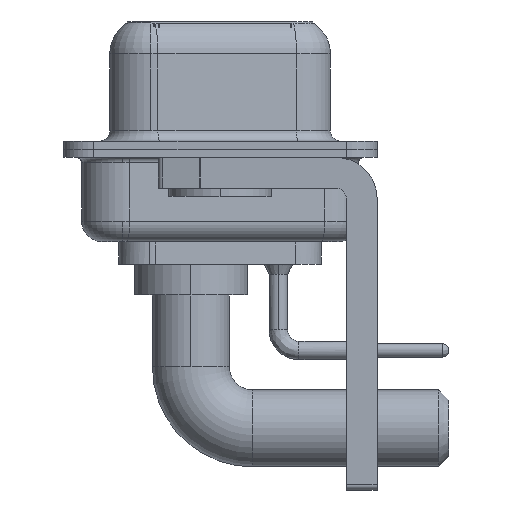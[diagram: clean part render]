
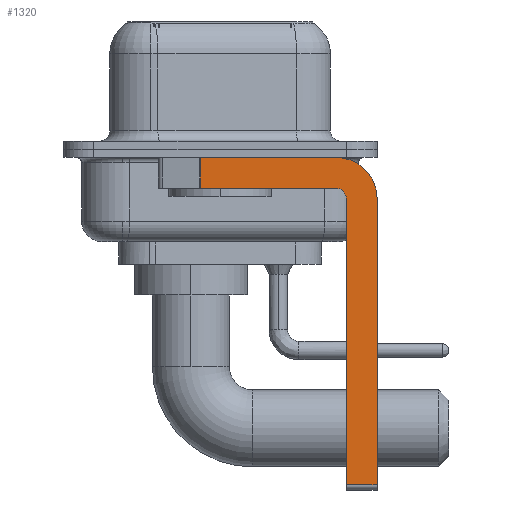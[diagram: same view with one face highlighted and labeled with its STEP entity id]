
A CAD part, left-side view. The second image highlights one B-rep face of the part: STEP entity #1320.
In plain terms, the highlighted planar face has unit normal (-1, 0, 0).
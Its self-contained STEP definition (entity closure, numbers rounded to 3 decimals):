
#208 = CARTESIAN_POINT ( 'NONE',  ( -2.9, 3., -0.4 ) ) ;
#1047 = AXIS2_PLACEMENT_3D ( 'NONE', #15279, #2071, #10603 ) ;
#1320 = ADVANCED_FACE ( 'NONE', ( #20540 ), #8215, .F. ) ;
#1343 = EDGE_CURVE ( 'NONE', #2158, #10176, #16879, .T. ) ;
#1547 = CARTESIAN_POINT ( 'NONE',  ( -2.9, -5.65, -2.4 ) ) ;
#1676 = DIRECTION ( 'NONE',  ( 0., -1., 0. ) ) ;
#2071 = DIRECTION ( 'NONE',  ( 1., 0., 0. ) ) ;
#2158 = VERTEX_POINT ( 'NONE', #21906 ) ;
#2584 = DIRECTION ( 'NONE',  ( 0., -1., 0. ) ) ;
#2932 = CARTESIAN_POINT ( 'NONE',  ( -2.9, -6.15, -2.4 ) ) ;
#2964 = CARTESIAN_POINT ( 'NONE',  ( -2.9, 0.978, -1.9 ) ) ;
#2982 = CARTESIAN_POINT ( 'NONE',  ( -2.9, 0.978, -1.9 ) ) ;
#3228 = VERTEX_POINT ( 'NONE', #15594 ) ;
#3400 = ORIENTED_EDGE ( 'NONE', *, *, #13802, .F. ) ;
#3750 = AXIS2_PLACEMENT_3D ( 'NONE', #1547, #20100, #18533 ) ;
#3889 = VECTOR ( 'NONE', #2584, 1000. ) ;
#4339 = VECTOR ( 'NONE', #12668, 1000. ) ;
#4344 = CARTESIAN_POINT ( 'NONE',  ( -2.9, -5.65, -1.9 ) ) ;
#4387 = VECTOR ( 'NONE', #21651, 1000. ) ;
#4644 = CARTESIAN_POINT ( 'NONE',  ( -2.9, -7.65, -2.4 ) ) ;
#4808 = ORIENTED_EDGE ( 'NONE', *, *, #9100, .F. ) ;
#4997 = CARTESIAN_POINT ( 'NONE',  ( -2.9, -5.65, -2.4 ) ) ;
#5145 = EDGE_CURVE ( 'NONE', #15355, #3228, #19470, .T. ) ;
#5320 = DIRECTION ( 'NONE',  ( 0., 0., -1. ) ) ;
#5697 = ORIENTED_EDGE ( 'NONE', *, *, #19944, .F. ) ;
#5735 = ORIENTED_EDGE ( 'NONE', *, *, #8685, .F. ) ;
#6081 = CARTESIAN_POINT ( 'NONE',  ( -2.9, -6.15, -16.35 ) ) ;
#6091 = VECTOR ( 'NONE', #7573, 1000. ) ;
#6569 = CARTESIAN_POINT ( 'NONE',  ( -2.9, -5.65, -0.4 ) ) ;
#6638 = VECTOR ( 'NONE', #1676, 1000. ) ;
#6986 = VERTEX_POINT ( 'NONE', #4344 ) ;
#7358 = LINE ( 'NONE', #4644, #6091 ) ;
#7573 = DIRECTION ( 'NONE',  ( 0., 0., -1. ) ) ;
#8215 = PLANE ( 'NONE',  #15480 ) ;
#8685 = EDGE_CURVE ( 'NONE', #10845, #3228, #7358, .T. ) ;
#9100 = EDGE_CURVE ( 'NONE', #15355, #11179, #9284, .T. ) ;
#9210 = LINE ( 'NONE', #15990, #4339 ) ;
#9284 = LINE ( 'NONE', #16064, #19599 ) ;
#10176 = VERTEX_POINT ( 'NONE', #6569 ) ;
#10603 = DIRECTION ( 'NONE',  ( 0., 0., -1. ) ) ;
#10845 = VERTEX_POINT ( 'NONE', #18503 ) ;
#11179 = VERTEX_POINT ( 'NONE', #2932 ) ;
#12248 = ORIENTED_EDGE ( 'NONE', *, *, #15546, .F. ) ;
#12668 = DIRECTION ( 'NONE',  ( 0., 1., 0. ) ) ;
#13802 = EDGE_CURVE ( 'NONE', #11179, #6986, #20790, .T. ) ;
#14986 = DIRECTION ( 'NONE',  ( 1., 0., 0. ) ) ;
#15279 = CARTESIAN_POINT ( 'NONE',  ( -2.9, -5.65, -2.4 ) ) ;
#15355 = VERTEX_POINT ( 'NONE', #6081 ) ;
#15480 = AXIS2_PLACEMENT_3D ( 'NONE', #4997, #14986, #5320 ) ;
#15506 = ORIENTED_EDGE ( 'NONE', *, *, #20907, .T. ) ;
#15546 = EDGE_CURVE ( 'NONE', #10176, #10845, #20439, .T. ) ;
#15594 = CARTESIAN_POINT ( 'NONE',  ( -2.9, -7.65, -16.35 ) ) ;
#15990 = CARTESIAN_POINT ( 'NONE',  ( -2.9, -5.65, -1.9 ) ) ;
#16064 = CARTESIAN_POINT ( 'NONE',  ( -2.9, -6.15, -16.6 ) ) ;
#16429 = ORIENTED_EDGE ( 'NONE', *, *, #5145, .T. ) ;
#16860 = EDGE_LOOP ( 'NONE', ( #19740, #15506, #5697, #3400, #4808, #16429, #5735, #12248 ) ) ;
#16879 = LINE ( 'NONE', #208, #6638 ) ;
#18503 = CARTESIAN_POINT ( 'NONE',  ( -2.9, -7.65, -2.4 ) ) ;
#18533 = DIRECTION ( 'NONE',  ( 0., 0., 1. ) ) ;
#19470 = LINE ( 'NONE', #21151, #3889 ) ;
#19599 = VECTOR ( 'NONE', #21414, 1000. ) ;
#19740 = ORIENTED_EDGE ( 'NONE', *, *, #1343, .F. ) ;
#19872 = LINE ( 'NONE', #2982, #4387 ) ;
#19944 = EDGE_CURVE ( 'NONE', #6986, #20519, #9210, .T. ) ;
#20100 = DIRECTION ( 'NONE',  ( -1., 0., 0. ) ) ;
#20439 = CIRCLE ( 'NONE', #1047, 2. ) ;
#20519 = VERTEX_POINT ( 'NONE', #2964 ) ;
#20540 = FACE_OUTER_BOUND ( 'NONE', #16860, .T. ) ;
#20790 = CIRCLE ( 'NONE', #3750, 0.5 ) ;
#20907 = EDGE_CURVE ( 'NONE', #2158, #20519, #19872, .T. ) ;
#21151 = CARTESIAN_POINT ( 'NONE',  ( -2.9, -5.65, -16.35 ) ) ;
#21414 = DIRECTION ( 'NONE',  ( 0., 0., 1. ) ) ;
#21651 = DIRECTION ( 'NONE',  ( 0., 0., -1. ) ) ;
#21906 = CARTESIAN_POINT ( 'NONE',  ( -2.9, 0.978, -0.4 ) ) ;
